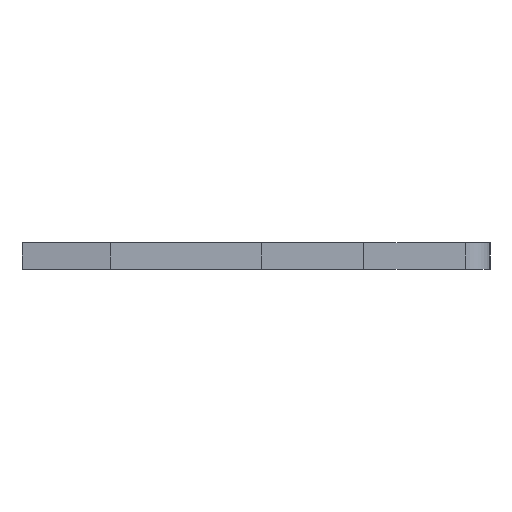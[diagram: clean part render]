
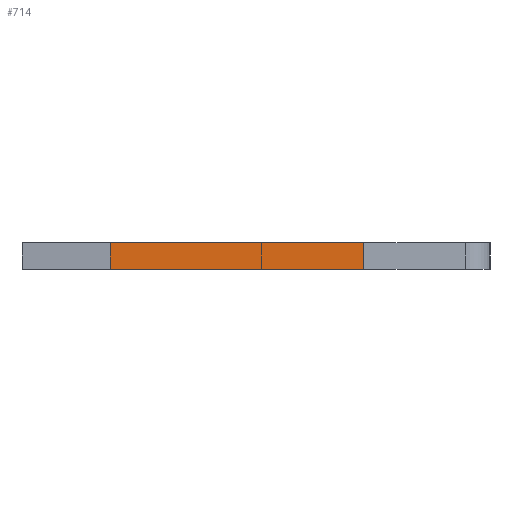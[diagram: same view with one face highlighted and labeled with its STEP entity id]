
A CAD part, left-side view. The second image highlights one B-rep face of the part: STEP entity #714.
In plain terms, the highlighted face is planar.
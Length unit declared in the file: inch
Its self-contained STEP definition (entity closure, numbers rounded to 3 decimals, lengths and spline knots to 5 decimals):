
#21 = VERTEX_POINT ( 'NONE', #535 ) ;
#178 = VECTOR ( 'NONE', #689, 39.37008 ) ;
#184 = DIRECTION ( 'NONE',  ( -1., 0., 0. ) ) ;
#251 = DIRECTION ( 'NONE',  ( 1., 0., 0. ) ) ;
#264 = VECTOR ( 'NONE', #895, 39.37008 ) ;
#309 = DIRECTION ( 'NONE',  ( 0., 1., 0. ) ) ;
#384 = CARTESIAN_POINT ( 'NONE',  ( 0.013, -0.099, -0.0575 ) ) ;
#535 = CARTESIAN_POINT ( 'NONE',  ( 0.013, -0.099, -0.0575 ) ) ;
#575 = AXIS2_PLACEMENT_3D ( 'NONE', #814, #614, #251 ) ;
#614 = DIRECTION ( 'NONE',  ( 0., 0., 1. ) ) ;
#689 = DIRECTION ( 'NONE',  ( -1., 0., 0. ) ) ;
#714 = ADVANCED_FACE ( 'NONE', ( #1729 ), #1361, .F. ) ;
#814 = CARTESIAN_POINT ( 'NONE',  ( 0.013, 0.146, -0.0575 ) ) ;
#895 = DIRECTION ( 'NONE',  ( 0., 1., 0. ) ) ;
#924 = EDGE_CURVE ( 'NONE', #1416, #1101, #2345, .T. ) ;
#956 = CARTESIAN_POINT ( 'NONE',  ( 0.013, 0.146, -0.0575 ) ) ;
#1010 = ORIENTED_EDGE ( 'NONE', *, *, #1653, .T. ) ;
#1051 = LINE ( 'NONE', #384, #1481 ) ;
#1101 = VERTEX_POINT ( 'NONE', #2171 ) ;
#1213 = CARTESIAN_POINT ( 'NONE',  ( -0.013, 0.146, -0.0575 ) ) ;
#1343 = LINE ( 'NONE', #1809, #178 ) ;
#1361 = PLANE ( 'NONE',  #575 ) ;
#1416 = VERTEX_POINT ( 'NONE', #1463 ) ;
#1463 = CARTESIAN_POINT ( 'NONE',  ( -0.013, -0.099, -0.0575 ) ) ;
#1465 = EDGE_CURVE ( 'NONE', #2288, #1101, #1343, .T. ) ;
#1481 = VECTOR ( 'NONE', #184, 39.37008 ) ;
#1492 = ORIENTED_EDGE ( 'NONE', *, *, #1541, .F. ) ;
#1541 = EDGE_CURVE ( 'NONE', #21, #2288, #2161, .T. ) ;
#1553 = EDGE_LOOP ( 'NONE', ( #2125, #1931, #1492, #1010 ) ) ;
#1653 = EDGE_CURVE ( 'NONE', #21, #1416, #1051, .T. ) ;
#1729 = FACE_OUTER_BOUND ( 'NONE', #1553, .T. ) ;
#1809 = CARTESIAN_POINT ( 'NONE',  ( 0.013, 0.146, -0.0575 ) ) ;
#1843 = VECTOR ( 'NONE', #309, 39.37008 ) ;
#1931 = ORIENTED_EDGE ( 'NONE', *, *, #1465, .F. ) ;
#2125 = ORIENTED_EDGE ( 'NONE', *, *, #924, .T. ) ;
#2161 = LINE ( 'NONE', #2308, #264 ) ;
#2171 = CARTESIAN_POINT ( 'NONE',  ( -0.013, 0.146, -0.0575 ) ) ;
#2288 = VERTEX_POINT ( 'NONE', #956 ) ;
#2308 = CARTESIAN_POINT ( 'NONE',  ( 0.013, 0.146, -0.0575 ) ) ;
#2345 = LINE ( 'NONE', #1213, #1843 ) ;
